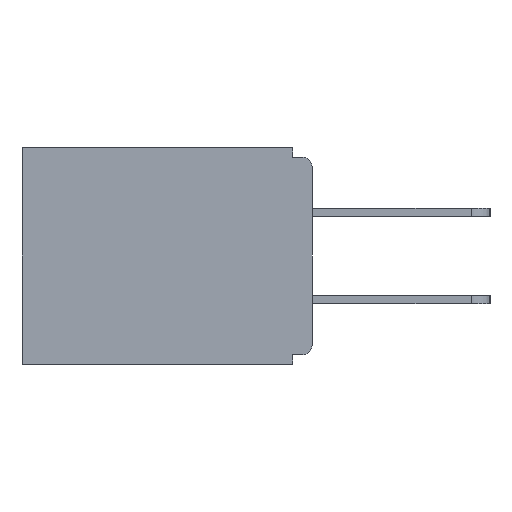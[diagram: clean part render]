
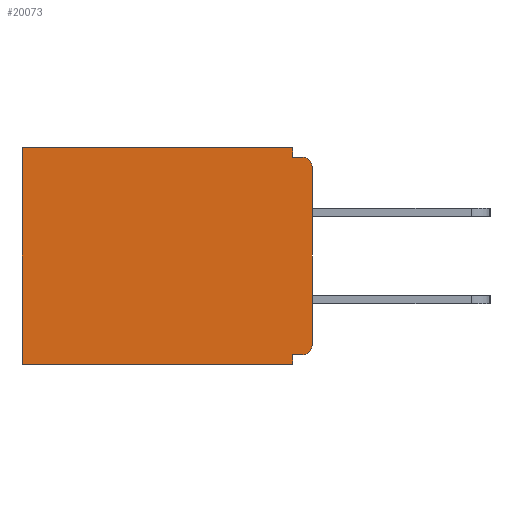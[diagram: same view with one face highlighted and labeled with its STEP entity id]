
A CAD part, left-side view. The second image highlights one B-rep face of the part: STEP entity #20073.
In plain terms, the highlighted planar face has unit normal (-1, 0, 0).
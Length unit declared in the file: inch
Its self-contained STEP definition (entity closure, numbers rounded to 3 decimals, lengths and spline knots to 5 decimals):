
#38 = LINE ( 'NONE', #10499, #18216 ) ;
#563 = CIRCLE ( 'NONE', #10270, 0.015 ) ;
#568 = LINE ( 'NONE', #720, #7846 ) ;
#698 = CARTESIAN_POINT ( 'NONE',  ( 0.298, 0.015, -0.328 ) ) ;
#720 = CARTESIAN_POINT ( 'NONE',  ( 0.298, 0.031, -0.343 ) ) ;
#934 = LINE ( 'NONE', #18008, #21309 ) ;
#1108 = CARTESIAN_POINT ( 'NONE',  ( 0.298, 0.015, -0.03 ) ) ;
#1303 = ORIENTED_EDGE ( 'NONE', *, *, #20839, .T. ) ;
#1347 = CARTESIAN_POINT ( 'NONE',  ( 0.298, 0., -0.313 ) ) ;
#1370 = CARTESIAN_POINT ( 'NONE',  ( 0.298, 0.46, -0.343 ) ) ;
#2134 = LINE ( 'NONE', #18758, #7472 ) ;
#2293 = VECTOR ( 'NONE', #10861, 39.37008 ) ;
#2841 = ORIENTED_EDGE ( 'NONE', *, *, #21462, .F. ) ;
#3060 = DIRECTION ( 'NONE',  ( 0., 0., -1. ) ) ;
#3105 = CARTESIAN_POINT ( 'NONE',  ( 0.298, 0., 0. ) ) ;
#3317 = EDGE_CURVE ( 'NONE', #6268, #16581, #8742, .T. ) ;
#3648 = ORIENTED_EDGE ( 'NONE', *, *, #15823, .T. ) ;
#4046 = CARTESIAN_POINT ( 'NONE',  ( 0.298, 0.031, 0. ) ) ;
#4379 = DIRECTION ( 'NONE',  ( 0., 0., -1. ) ) ;
#4445 = DIRECTION ( 'NONE',  ( 0., 0., -1. ) ) ;
#4549 = DIRECTION ( 'NONE',  ( -1., 0., 0. ) ) ;
#4569 = FACE_OUTER_BOUND ( 'NONE', #7592, .T. ) ;
#4938 = CIRCLE ( 'NONE', #19242, 0.015 ) ;
#5422 = ORIENTED_EDGE ( 'NONE', *, *, #19643, .F. ) ;
#5480 = VERTEX_POINT ( 'NONE', #15957 ) ;
#6057 = VERTEX_POINT ( 'NONE', #4046 ) ;
#6268 = VERTEX_POINT ( 'NONE', #698 ) ;
#6490 = CARTESIAN_POINT ( 'NONE',  ( 0.298, 0.031, -0.343 ) ) ;
#6617 = ORIENTED_EDGE ( 'NONE', *, *, #13240, .F. ) ;
#7348 = LINE ( 'NONE', #19154, #21003 ) ;
#7418 = VECTOR ( 'NONE', #20593, 39.37008 ) ;
#7472 = VECTOR ( 'NONE', #20385, 39.37008 ) ;
#7553 = CARTESIAN_POINT ( 'NONE',  ( 0.298, 0.015, -0.313 ) ) ;
#7592 = EDGE_LOOP ( 'NONE', ( #15070, #15709, #2841, #3648, #1303, #6617, #14248, #14108, #17472, #5422 ) ) ;
#7831 = CARTESIAN_POINT ( 'NONE',  ( 0.298, 0.031, -0.328 ) ) ;
#7846 = VECTOR ( 'NONE', #4379, 39.37008 ) ;
#8460 = VERTEX_POINT ( 'NONE', #18978 ) ;
#8742 = LINE ( 'NONE', #12582, #2293 ) ;
#9412 = DIRECTION ( 'NONE',  ( 0., 0., -1. ) ) ;
#9560 = EDGE_CURVE ( 'NONE', #16581, #16530, #568, .T. ) ;
#10026 = VERTEX_POINT ( 'NONE', #22998 ) ;
#10270 = AXIS2_PLACEMENT_3D ( 'NONE', #1108, #4549, #15414 ) ;
#10499 = CARTESIAN_POINT ( 'NONE',  ( 0.298, 0., -0.015 ) ) ;
#10861 = DIRECTION ( 'NONE',  ( 0., 1., 0. ) ) ;
#11702 = CARTESIAN_POINT ( 'NONE',  ( 0.298, 0., 0. ) ) ;
#12582 = CARTESIAN_POINT ( 'NONE',  ( 0.298, 0., -0.328 ) ) ;
#12903 = LINE ( 'NONE', #6490, #20413 ) ;
#13064 = CARTESIAN_POINT ( 'NONE',  ( 0.298, 0.031, -0.343 ) ) ;
#13164 = EDGE_CURVE ( 'NONE', #6268, #20849, #4938, .T. ) ;
#13240 = EDGE_CURVE ( 'NONE', #16530, #21978, #2134, .T. ) ;
#14010 = DIRECTION ( 'NONE',  ( 0., -1., 0. ) ) ;
#14108 = ORIENTED_EDGE ( 'NONE', *, *, #3317, .F. ) ;
#14248 = ORIENTED_EDGE ( 'NONE', *, *, #9560, .F. ) ;
#14513 = DIRECTION ( 'NONE',  ( 0., 1., 0. ) ) ;
#15070 = ORIENTED_EDGE ( 'NONE', *, *, #22458, .T. ) ;
#15290 = PLANE ( 'NONE',  #19775 ) ;
#15414 = DIRECTION ( 'NONE',  ( 0., 0., -1. ) ) ;
#15709 = ORIENTED_EDGE ( 'NONE', *, *, #20918, .F. ) ;
#15823 = EDGE_CURVE ( 'NONE', #6057, #5480, #934, .T. ) ;
#15957 = CARTESIAN_POINT ( 'NONE',  ( 0.298, 0.46, 0. ) ) ;
#16530 = VERTEX_POINT ( 'NONE', #13064 ) ;
#16581 = VERTEX_POINT ( 'NONE', #7831 ) ;
#16925 = DIRECTION ( 'NONE',  ( 1., 0., 0. ) ) ;
#17472 = ORIENTED_EDGE ( 'NONE', *, *, #13164, .T. ) ;
#18008 = CARTESIAN_POINT ( 'NONE',  ( 0.298, 0., 0. ) ) ;
#18216 = VECTOR ( 'NONE', #14010, 39.37008 ) ;
#18758 = CARTESIAN_POINT ( 'NONE',  ( 0.298, 0., -0.343 ) ) ;
#18978 = CARTESIAN_POINT ( 'NONE',  ( 0.298, 0.031, -0.015 ) ) ;
#19087 = CARTESIAN_POINT ( 'NONE',  ( 0.298, 0.015, -0.015 ) ) ;
#19154 = CARTESIAN_POINT ( 'NONE',  ( 0.298, 0.46, 0. ) ) ;
#19242 = AXIS2_PLACEMENT_3D ( 'NONE', #7553, #21807, #9412 ) ;
#19643 = EDGE_CURVE ( 'NONE', #10026, #20849, #21340, .T. ) ;
#19775 = AXIS2_PLACEMENT_3D ( 'NONE', #11702, #16925, #22297 ) ;
#20073 = ADVANCED_FACE ( 'NONE', ( #4569 ), #15290, .F. ) ;
#20170 = VERTEX_POINT ( 'NONE', #19087 ) ;
#20385 = DIRECTION ( 'NONE',  ( 0., 1., 0. ) ) ;
#20413 = VECTOR ( 'NONE', #4445, 39.37008 ) ;
#20593 = DIRECTION ( 'NONE',  ( 0., 0., -1. ) ) ;
#20839 = EDGE_CURVE ( 'NONE', #5480, #21978, #7348, .T. ) ;
#20849 = VERTEX_POINT ( 'NONE', #1347 ) ;
#20918 = EDGE_CURVE ( 'NONE', #8460, #20170, #38, .T. ) ;
#21003 = VECTOR ( 'NONE', #3060, 39.37008 ) ;
#21309 = VECTOR ( 'NONE', #14513, 39.37008 ) ;
#21340 = LINE ( 'NONE', #3105, #7418 ) ;
#21462 = EDGE_CURVE ( 'NONE', #6057, #8460, #12903, .T. ) ;
#21807 = DIRECTION ( 'NONE',  ( -1., 0., 0. ) ) ;
#21978 = VERTEX_POINT ( 'NONE', #1370 ) ;
#22297 = DIRECTION ( 'NONE',  ( 0., 0., -1. ) ) ;
#22458 = EDGE_CURVE ( 'NONE', #10026, #20170, #563, .T. ) ;
#22998 = CARTESIAN_POINT ( 'NONE',  ( 0.298, 0., -0.03 ) ) ;
